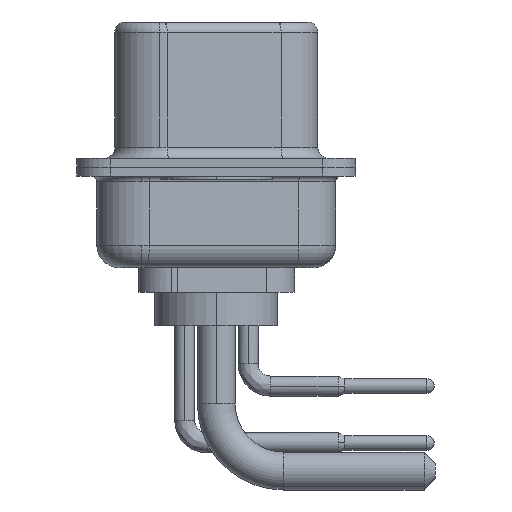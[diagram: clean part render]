
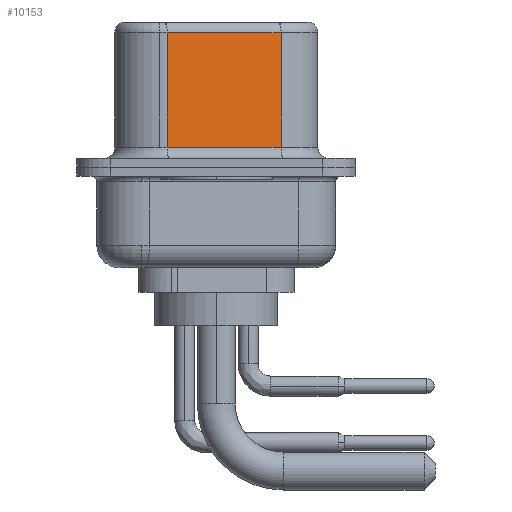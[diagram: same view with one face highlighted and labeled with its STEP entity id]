
A CAD part, left-side view. The second image highlights one B-rep face of the part: STEP entity #10153.
In plain terms, the highlighted planar face has unit normal (-0.985, -0.174, 0).
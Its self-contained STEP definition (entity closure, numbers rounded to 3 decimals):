
#631 = CARTESIAN_POINT ( 'NONE',  ( 4.58, -2.897, 0.9 ) ) ;
#781 = EDGE_LOOP ( 'NONE', ( #5460, #11523, #19904, #23683 ) ) ;
#1436 = EDGE_CURVE ( 'NONE', #8742, #26075, #5608, .T. ) ;
#2235 = VECTOR ( 'NONE', #16565, 1000. ) ;
#2618 = EDGE_CURVE ( 'NONE', #18054, #16714, #19837, .T. ) ;
#3300 = CARTESIAN_POINT ( 'NONE',  ( 4.58, -2.897, 6.02 ) ) ;
#3527 = PLANE ( 'NONE',  #5727 ) ;
#4221 = CARTESIAN_POINT ( 'NONE',  ( 4.58, -2.897, 6.52 ) ) ;
#4259 = VECTOR ( 'NONE', #26090, 1000. ) ;
#5460 = ORIENTED_EDGE ( 'NONE', *, *, #15505, .F. ) ;
#5608 = LINE ( 'NONE', #3300, #23972 ) ;
#5727 = AXIS2_PLACEMENT_3D ( 'NONE', #26517, #5960, #22348 ) ;
#5927 = LINE ( 'NONE', #20555, #4259 ) ;
#5960 = DIRECTION ( 'NONE',  ( 0.985, 0.174, 0. ) ) ;
#8742 = VERTEX_POINT ( 'NONE', #8784 ) ;
#8784 = CARTESIAN_POINT ( 'NONE',  ( 4.58, -2.897, 6.02 ) ) ;
#9544 = CARTESIAN_POINT ( 'NONE',  ( 4.58, -2.897, 0.9 ) ) ;
#10153 = ADVANCED_FACE ( 'NONE', ( #13977 ), #3527, .F. ) ;
#10723 = CARTESIAN_POINT ( 'NONE',  ( 3.68, 2.203, 0.9 ) ) ;
#11523 = ORIENTED_EDGE ( 'NONE', *, *, #1436, .T. ) ;
#11721 = DIRECTION ( 'NONE',  ( -0.174, 0.985, 0. ) ) ;
#11936 = EDGE_CURVE ( 'NONE', #26075, #18054, #5927, .T. ) ;
#13977 = FACE_OUTER_BOUND ( 'NONE', #781, .T. ) ;
#15505 = EDGE_CURVE ( 'NONE', #8742, #16714, #20347, .T. ) ;
#16565 = DIRECTION ( 'NONE',  ( 0., 0., -1. ) ) ;
#16714 = VERTEX_POINT ( 'NONE', #631 ) ;
#18054 = VERTEX_POINT ( 'NONE', #10723 ) ;
#19837 = LINE ( 'NONE', #9544, #25304 ) ;
#19904 = ORIENTED_EDGE ( 'NONE', *, *, #11936, .T. ) ;
#20347 = LINE ( 'NONE', #4221, #2235 ) ;
#20372 = DIRECTION ( 'NONE',  ( 0.174, -0.985, 0. ) ) ;
#20555 = CARTESIAN_POINT ( 'NONE',  ( 3.68, 2.203, 6.52 ) ) ;
#22348 = DIRECTION ( 'NONE',  ( -0.174, 0.985, 0. ) ) ;
#23474 = CARTESIAN_POINT ( 'NONE',  ( 3.68, 2.203, 6.02 ) ) ;
#23683 = ORIENTED_EDGE ( 'NONE', *, *, #2618, .T. ) ;
#23972 = VECTOR ( 'NONE', #11721, 1000. ) ;
#25304 = VECTOR ( 'NONE', #20372, 1000. ) ;
#26075 = VERTEX_POINT ( 'NONE', #23474 ) ;
#26090 = DIRECTION ( 'NONE',  ( 0., 0., -1. ) ) ;
#26517 = CARTESIAN_POINT ( 'NONE',  ( 4.58, -2.897, 6.52 ) ) ;
